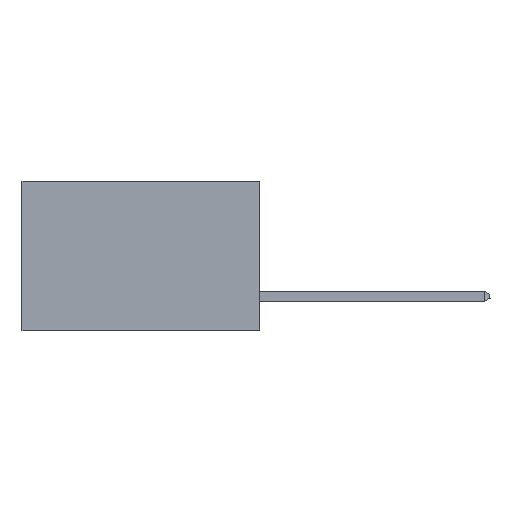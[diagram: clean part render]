
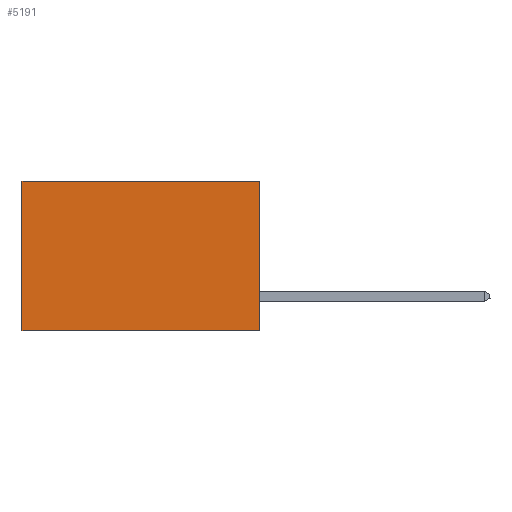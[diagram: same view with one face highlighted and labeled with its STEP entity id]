
A CAD part, left-side view. The second image highlights one B-rep face of the part: STEP entity #5191.
In plain terms, the highlighted planar face has unit normal (-1, 0, 0).
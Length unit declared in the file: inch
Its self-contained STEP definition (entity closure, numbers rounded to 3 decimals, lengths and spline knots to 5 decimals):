
#557 = VECTOR ( 'NONE', #15113, 39.37008 ) ;
#1109 = VERTEX_POINT ( 'NONE', #24935 ) ;
#1222 = DIRECTION ( 'NONE',  ( 0., 1., 0. ) ) ;
#1348 = LINE ( 'NONE', #29670, #557 ) ;
#2647 = FACE_OUTER_BOUND ( 'NONE', #31487, .T. ) ;
#4230 = VERTEX_POINT ( 'NONE', #30247 ) ;
#4247 = EDGE_CURVE ( 'NONE', #1109, #7450, #6133, .T. ) ;
#4987 = VECTOR ( 'NONE', #23277, 39.37008 ) ;
#5191 = ADVANCED_FACE ( 'NONE', ( #2647 ), #27313, .F. ) ;
#5813 = ORIENTED_EDGE ( 'NONE', *, *, #22751, .F. ) ;
#6133 = LINE ( 'NONE', #19581, #25621 ) ;
#7450 = VERTEX_POINT ( 'NONE', #14989 ) ;
#9268 = VECTOR ( 'NONE', #1222, 39.37008 ) ;
#13605 = AXIS2_PLACEMENT_3D ( 'NONE', #27352, #27453, #27178 ) ;
#13683 = CARTESIAN_POINT ( 'NONE',  ( 0.277, 0.59, -0.37 ) ) ;
#14989 = CARTESIAN_POINT ( 'NONE',  ( 0.277, 0., -0.37 ) ) ;
#15113 = DIRECTION ( 'NONE',  ( 0., 1., 0. ) ) ;
#15631 = ORIENTED_EDGE ( 'NONE', *, *, #17341, .T. ) ;
#17341 = EDGE_CURVE ( 'NONE', #1109, #4230, #27946, .T. ) ;
#18135 = ORIENTED_EDGE ( 'NONE', *, *, #28392, .T. ) ;
#18376 = CARTESIAN_POINT ( 'NONE',  ( 0.277, 0., 0. ) ) ;
#18696 = DIRECTION ( 'NONE',  ( 0., 0., -1. ) ) ;
#19581 = CARTESIAN_POINT ( 'NONE',  ( 0.277, 0., -0.37 ) ) ;
#22751 = EDGE_CURVE ( 'NONE', #7450, #27276, #1348, .T. ) ;
#22975 = LINE ( 'NONE', #13683, #4987 ) ;
#23277 = DIRECTION ( 'NONE',  ( 0., 0., -1. ) ) ;
#24935 = CARTESIAN_POINT ( 'NONE',  ( 0.277, 0., 0. ) ) ;
#25014 = ORIENTED_EDGE ( 'NONE', *, *, #4247, .F. ) ;
#25621 = VECTOR ( 'NONE', #18696, 39.37008 ) ;
#26744 = CARTESIAN_POINT ( 'NONE',  ( 0.277, 0.59, -0.37 ) ) ;
#27178 = DIRECTION ( 'NONE',  ( 0., 0., -1. ) ) ;
#27276 = VERTEX_POINT ( 'NONE', #26744 ) ;
#27313 = PLANE ( 'NONE',  #13605 ) ;
#27352 = CARTESIAN_POINT ( 'NONE',  ( 0.277, 0., -0.37 ) ) ;
#27453 = DIRECTION ( 'NONE',  ( 1., 0., 0. ) ) ;
#27946 = LINE ( 'NONE', #18376, #9268 ) ;
#28392 = EDGE_CURVE ( 'NONE', #4230, #27276, #22975, .T. ) ;
#29670 = CARTESIAN_POINT ( 'NONE',  ( 0.277, 0., -0.37 ) ) ;
#30247 = CARTESIAN_POINT ( 'NONE',  ( 0.277, 0.59, 0. ) ) ;
#31487 = EDGE_LOOP ( 'NONE', ( #18135, #5813, #25014, #15631 ) ) ;
